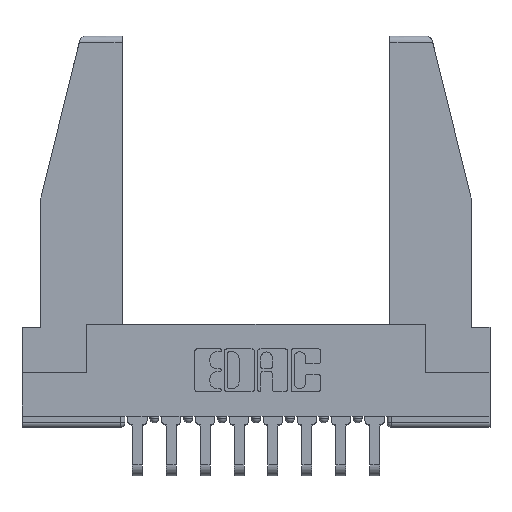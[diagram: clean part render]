
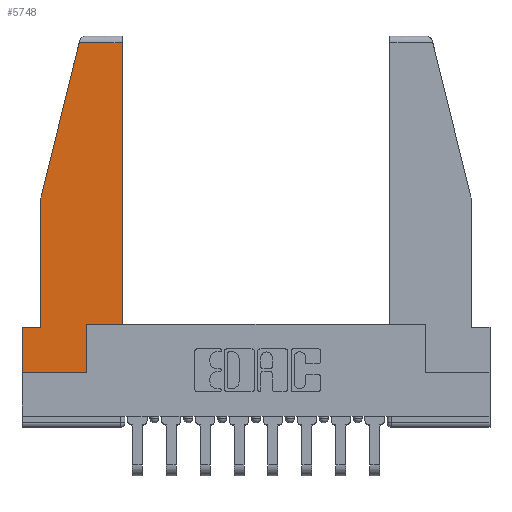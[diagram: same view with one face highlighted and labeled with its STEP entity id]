
A CAD part, top view. The second image highlights one B-rep face of the part: STEP entity #5748.
In plain terms, the highlighted planar face has unit normal (0, 0, 1).
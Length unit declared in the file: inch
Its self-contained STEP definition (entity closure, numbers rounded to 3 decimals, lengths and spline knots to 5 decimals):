
#103 = ORIENTED_EDGE ( 'NONE', *, *, #6098, .T. ) ;
#389 = CARTESIAN_POINT ( 'NONE',  ( 0., 0., 0. ) ) ;
#536 = VERTEX_POINT ( 'NONE', #5464 ) ;
#625 = CARTESIAN_POINT ( 'NONE',  ( 0., 0., 0. ) ) ;
#888 = CARTESIAN_POINT ( 'NONE',  ( 0., 0., 0. ) ) ;
#1057 = VERTEX_POINT ( 'NONE', #888 ) ;
#1181 = LINE ( 'NONE', #10572, #12352 ) ;
#1393 = PLANE ( 'NONE',  #10516 ) ;
#1498 = EDGE_CURVE ( 'NONE', #536, #7185, #2225, .T. ) ;
#1829 = ORIENTED_EDGE ( 'NONE', *, *, #6314, .T. ) ;
#1940 = ORIENTED_EDGE ( 'NONE', *, *, #8288, .T. ) ;
#1968 = CARTESIAN_POINT ( 'NONE',  ( 0.461, 0.223, 0. ) ) ;
#2144 = EDGE_CURVE ( 'NONE', #13836, #536, #5208, .T. ) ;
#2199 = CARTESIAN_POINT ( 'NONE',  ( 0.2636, 1.52, 0. ) ) ;
#2225 = LINE ( 'NONE', #3311, #11280 ) ;
#2370 = VERTEX_POINT ( 'NONE', #11499 ) ;
#2735 = CARTESIAN_POINT ( 'NONE',  ( 0.271, 1.55, 0. ) ) ;
#2776 = VECTOR ( 'NONE', #13920, 39.37008 ) ;
#3183 = DIRECTION ( 'NONE',  ( 0., 1., 0. ) ) ;
#3287 = CARTESIAN_POINT ( 'NONE',  ( 0., 0.21, 0. ) ) ;
#3311 = CARTESIAN_POINT ( 'NONE',  ( 0.086, 0.8, 0. ) ) ;
#3377 = CARTESIAN_POINT ( 'NONE',  ( 0., 1.52, 0. ) ) ;
#3389 = VERTEX_POINT ( 'NONE', #12846 ) ;
#3613 = DIRECTION ( 'NONE',  ( -1., 0., 0. ) ) ;
#3704 = VECTOR ( 'NONE', #14643, 39.37008 ) ;
#3710 = DIRECTION ( 'NONE',  ( 0., 0., 1. ) ) ;
#3760 = CARTESIAN_POINT ( 'NONE',  ( 0.297, 0.223, 0. ) ) ;
#3999 = DIRECTION ( 'NONE',  ( 1., 0., 0. ) ) ;
#4044 = EDGE_CURVE ( 'NONE', #9338, #2370, #10035, .T. ) ;
#4143 = ORIENTED_EDGE ( 'NONE', *, *, #10761, .T. ) ;
#4696 = LINE ( 'NONE', #3377, #6970 ) ;
#5152 = ORIENTED_EDGE ( 'NONE', *, *, #11565, .T. ) ;
#5208 = LINE ( 'NONE', #2735, #8572 ) ;
#5385 = VERTEX_POINT ( 'NONE', #13354 ) ;
#5464 = CARTESIAN_POINT ( 'NONE',  ( 0.086, 0.8, 0. ) ) ;
#5506 = LINE ( 'NONE', #6812, #8462 ) ;
#5748 = ADVANCED_FACE ( 'NONE', ( #9848 ), #1393, .T. ) ;
#5813 = DIRECTION ( 'NONE',  ( 0., -1., 0. ) ) ;
#6098 = EDGE_CURVE ( 'NONE', #2370, #6338, #14107, .T. ) ;
#6314 = EDGE_CURVE ( 'NONE', #7185, #5385, #6602, .T. ) ;
#6338 = VERTEX_POINT ( 'NONE', #1968 ) ;
#6384 = CARTESIAN_POINT ( 'NONE',  ( 0.297, 0., 0. ) ) ;
#6602 = LINE ( 'NONE', #3287, #2776 ) ;
#6812 = CARTESIAN_POINT ( 'NONE',  ( 0.461, 0.223, 0. ) ) ;
#6970 = VECTOR ( 'NONE', #3613, 39.37008 ) ;
#7185 = VERTEX_POINT ( 'NONE', #9723 ) ;
#8009 = DIRECTION ( 'NONE',  ( 0., -1., 0. ) ) ;
#8288 = EDGE_CURVE ( 'NONE', #5385, #1057, #1181, .T. ) ;
#8324 = EDGE_LOOP ( 'NONE', ( #5152, #4143, #8769, #11818, #1829, #1940, #10166, #11882, #103 ) ) ;
#8372 = DIRECTION ( 'NONE',  ( 1., 0., 0. ) ) ;
#8462 = VECTOR ( 'NONE', #3183, 39.37008 ) ;
#8572 = VECTOR ( 'NONE', #13438, 39.37008 ) ;
#8769 = ORIENTED_EDGE ( 'NONE', *, *, #2144, .T. ) ;
#9338 = VERTEX_POINT ( 'NONE', #6384 ) ;
#9723 = CARTESIAN_POINT ( 'NONE',  ( 0.086, 0.21, 0. ) ) ;
#9848 = FACE_OUTER_BOUND ( 'NONE', #8324, .T. ) ;
#10035 = LINE ( 'NONE', #14960, #14952 ) ;
#10166 = ORIENTED_EDGE ( 'NONE', *, *, #14284, .T. ) ;
#10516 = AXIS2_PLACEMENT_3D ( 'NONE', #625, #3710, #3999 ) ;
#10572 = CARTESIAN_POINT ( 'NONE',  ( 0., 0.21, 0. ) ) ;
#10761 = EDGE_CURVE ( 'NONE', #3389, #13836, #4696, .T. ) ;
#11280 = VECTOR ( 'NONE', #8009, 39.37008 ) ;
#11499 = CARTESIAN_POINT ( 'NONE',  ( 0.297, 0.223, 0. ) ) ;
#11565 = EDGE_CURVE ( 'NONE', #6338, #3389, #5506, .T. ) ;
#11818 = ORIENTED_EDGE ( 'NONE', *, *, #1498, .T. ) ;
#11882 = ORIENTED_EDGE ( 'NONE', *, *, #4044, .T. ) ;
#12352 = VECTOR ( 'NONE', #5813, 39.37008 ) ;
#12654 = DIRECTION ( 'NONE',  ( 0., 1., 0. ) ) ;
#12846 = CARTESIAN_POINT ( 'NONE',  ( 0.461, 1.52, 0. ) ) ;
#12961 = LINE ( 'NONE', #389, #3704 ) ;
#13354 = CARTESIAN_POINT ( 'NONE',  ( 0., 0.21, 0. ) ) ;
#13438 = DIRECTION ( 'NONE',  ( -0.239, -0.971, 0. ) ) ;
#13456 = VECTOR ( 'NONE', #8372, 39.37008 ) ;
#13836 = VERTEX_POINT ( 'NONE', #2199 ) ;
#13920 = DIRECTION ( 'NONE',  ( -1., 0., 0. ) ) ;
#14107 = LINE ( 'NONE', #3760, #13456 ) ;
#14284 = EDGE_CURVE ( 'NONE', #1057, #9338, #12961, .T. ) ;
#14643 = DIRECTION ( 'NONE',  ( 1., 0., 0. ) ) ;
#14952 = VECTOR ( 'NONE', #12654, 39.37008 ) ;
#14960 = CARTESIAN_POINT ( 'NONE',  ( 0.297, 0., 0. ) ) ;
